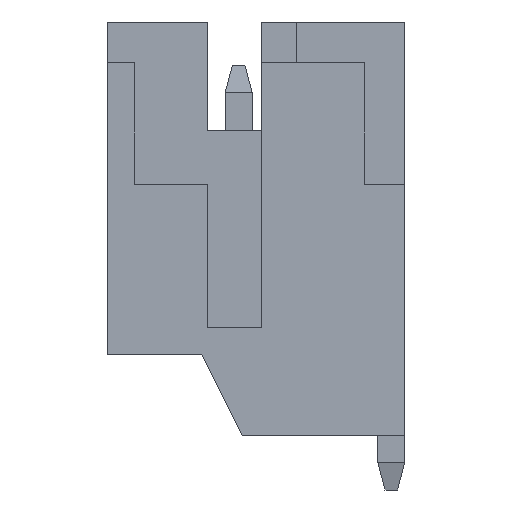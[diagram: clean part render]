
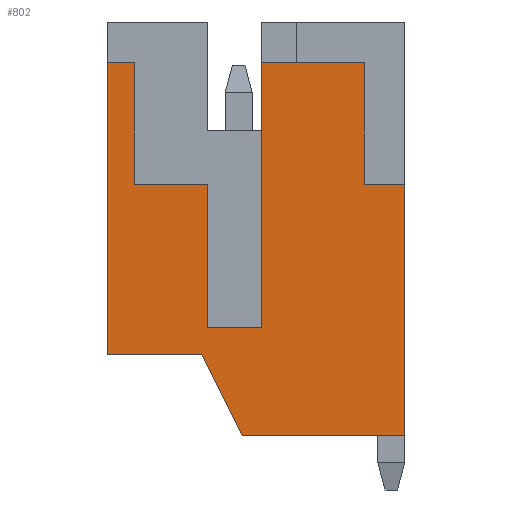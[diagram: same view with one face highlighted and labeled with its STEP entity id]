
A CAD part, left-side view. The second image highlights one B-rep face of the part: STEP entity #802.
In plain terms, the highlighted planar face has unit normal (-1, 0, 0).
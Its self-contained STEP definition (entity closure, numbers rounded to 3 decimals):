
#33 = LINE ( 'NONE', #486, #3350 ) ;
#57 = ORIENTED_EDGE ( 'NONE', *, *, #818, .F. ) ;
#66 = LINE ( 'NONE', #4594, #2860 ) ;
#202 = CARTESIAN_POINT ( 'NONE',  ( -3., 1.93, 5.4 ) ) ;
#237 = EDGE_LOOP ( 'NONE', ( #774, #1345, #1196, #2845, #3341, #2224, #549, #3415, #449, #1396, #1850, #57, #3068, #2094 ) ) ;
#280 = LINE ( 'NONE', #2753, #3090 ) ;
#297 = VERTEX_POINT ( 'NONE', #1133 ) ;
#317 = PLANE ( 'NONE',  #3844 ) ;
#449 = ORIENTED_EDGE ( 'NONE', *, *, #2692, .T. ) ;
#486 = CARTESIAN_POINT ( 'NONE',  ( -3., -0.42, 3.15 ) ) ;
#506 = EDGE_CURVE ( 'NONE', #2816, #3251, #66, .T. ) ;
#549 = ORIENTED_EDGE ( 'NONE', *, *, #1288, .F. ) ;
#567 = EDGE_CURVE ( 'NONE', #297, #2436, #4172, .T. ) ;
#638 = VERTEX_POINT ( 'NONE', #2404 ) ;
#639 = DIRECTION ( 'NONE',  ( 0., -1., 0. ) ) ;
#677 = VERTEX_POINT ( 'NONE', #3921 ) ;
#688 = EDGE_CURVE ( 'NONE', #4280, #1674, #4513, .T. ) ;
#707 = VERTEX_POINT ( 'NONE', #3937 ) ;
#709 = CARTESIAN_POINT ( 'NONE',  ( -3., 0.68, 0. ) ) ;
#731 = DIRECTION ( 'NONE',  ( -1., 0., 0. ) ) ;
#774 = ORIENTED_EDGE ( 'NONE', *, *, #688, .T. ) ;
#795 = VECTOR ( 'NONE', #3804, 1000. ) ;
#802 = ADVANCED_FACE ( 'NONE', ( #1606 ), #317, .T. ) ;
#818 = EDGE_CURVE ( 'NONE', #2758, #677, #2747, .T. ) ;
#819 = VERTEX_POINT ( 'NONE', #4716 ) ;
#901 = DIRECTION ( 'NONE',  ( 0., 0., 1. ) ) ;
#972 = LINE ( 'NONE', #1584, #1324 ) ;
#1048 = CARTESIAN_POINT ( 'NONE',  ( -3., -3.07, 5.4 ) ) ;
#1133 = CARTESIAN_POINT ( 'NONE',  ( -3., -0.42, 5.4 ) ) ;
#1196 = ORIENTED_EDGE ( 'NONE', *, *, #1969, .T. ) ;
#1211 = VECTOR ( 'NONE', #2180, 1000. ) ;
#1288 = EDGE_CURVE ( 'NONE', #819, #3251, #2928, .T. ) ;
#1324 = VECTOR ( 'NONE', #1973, 1000. ) ;
#1335 = CARTESIAN_POINT ( 'NONE',  ( -3., -3.07, -1.5 ) ) ;
#1345 = ORIENTED_EDGE ( 'NONE', *, *, #2744, .T. ) ;
#1355 = VERTEX_POINT ( 'NONE', #3945 ) ;
#1380 = DIRECTION ( 'NONE',  ( 0., 1., 0. ) ) ;
#1396 = ORIENTED_EDGE ( 'NONE', *, *, #567, .T. ) ;
#1452 = CARTESIAN_POINT ( 'NONE',  ( -3., -0.42, 0.5 ) ) ;
#1479 = CARTESIAN_POINT ( 'NONE',  ( -3., 0.58, 3.15 ) ) ;
#1492 = DIRECTION ( 'NONE',  ( 0., 0., 1. ) ) ;
#1498 = VECTOR ( 'NONE', #4451, 1000. ) ;
#1584 = CARTESIAN_POINT ( 'NONE',  ( -3., -0.42, 0.5 ) ) ;
#1606 = FACE_OUTER_BOUND ( 'NONE', #237, .T. ) ;
#1674 = VERTEX_POINT ( 'NONE', #3784 ) ;
#1850 = ORIENTED_EDGE ( 'NONE', *, *, #2084, .F. ) ;
#1875 = VERTEX_POINT ( 'NONE', #709 ) ;
#1893 = EDGE_CURVE ( 'NONE', #707, #4280, #1959, .T. ) ;
#1898 = LINE ( 'NONE', #2976, #1498 ) ;
#1899 = EDGE_CURVE ( 'NONE', #1875, #638, #1898, .T. ) ;
#1959 = LINE ( 'NONE', #3677, #2855 ) ;
#1969 = EDGE_CURVE ( 'NONE', #1355, #1875, #2918, .T. ) ;
#1973 = DIRECTION ( 'NONE',  ( 0., -1., 0. ) ) ;
#1994 = EDGE_CURVE ( 'NONE', #819, #2761, #2241, .T. ) ;
#2038 = DIRECTION ( 'NONE',  ( 0., -1., 0. ) ) ;
#2072 = VECTOR ( 'NONE', #2038, 1000. ) ;
#2084 = EDGE_CURVE ( 'NONE', #677, #2436, #972, .T. ) ;
#2094 = ORIENTED_EDGE ( 'NONE', *, *, #1893, .T. ) ;
#2165 = EDGE_CURVE ( 'NONE', #638, #2816, #3093, .T. ) ;
#2180 = DIRECTION ( 'NONE',  ( 0., 0., -1. ) ) ;
#2191 = VECTOR ( 'NONE', #639, 1000. ) ;
#2224 = ORIENTED_EDGE ( 'NONE', *, *, #506, .T. ) ;
#2231 = LINE ( 'NONE', #2748, #795 ) ;
#2241 = LINE ( 'NONE', #2259, #4057 ) ;
#2259 = CARTESIAN_POINT ( 'NONE',  ( -3., -2.32, 3.15 ) ) ;
#2404 = CARTESIAN_POINT ( 'NONE',  ( -3., -0.07, -1.5 ) ) ;
#2436 = VERTEX_POINT ( 'NONE', #1452 ) ;
#2692 = EDGE_CURVE ( 'NONE', #2761, #297, #2231, .T. ) ;
#2744 = EDGE_CURVE ( 'NONE', #1674, #1355, #280, .T. ) ;
#2747 = LINE ( 'NONE', #1479, #1211 ) ;
#2748 = CARTESIAN_POINT ( 'NONE',  ( -3., -3.07, 5.4 ) ) ;
#2753 = CARTESIAN_POINT ( 'NONE',  ( -3., 2.43, 6.15 ) ) ;
#2758 = VERTEX_POINT ( 'NONE', #2919 ) ;
#2761 = VERTEX_POINT ( 'NONE', #4618 ) ;
#2807 = DIRECTION ( 'NONE',  ( 0., 0., -1. ) ) ;
#2816 = VERTEX_POINT ( 'NONE', #1335 ) ;
#2829 = CARTESIAN_POINT ( 'NONE',  ( -3., -2.32, 3.15 ) ) ;
#2845 = ORIENTED_EDGE ( 'NONE', *, *, #1899, .T. ) ;
#2855 = VECTOR ( 'NONE', #1492, 1000. ) ;
#2860 = VECTOR ( 'NONE', #901, 1000. ) ;
#2918 = LINE ( 'NONE', #2954, #3208 ) ;
#2919 = CARTESIAN_POINT ( 'NONE',  ( -3., 0.58, 3.15 ) ) ;
#2928 = LINE ( 'NONE', #2829, #2191 ) ;
#2954 = CARTESIAN_POINT ( 'NONE',  ( -3., 2.43, 0. ) ) ;
#2976 = CARTESIAN_POINT ( 'NONE',  ( -3., -0.07, -1.5 ) ) ;
#3068 = ORIENTED_EDGE ( 'NONE', *, *, #4084, .F. ) ;
#3090 = VECTOR ( 'NONE', #2807, 1000. ) ;
#3093 = LINE ( 'NONE', #4254, #2072 ) ;
#3208 = VECTOR ( 'NONE', #3699, 1000. ) ;
#3251 = VERTEX_POINT ( 'NONE', #4030 ) ;
#3341 = ORIENTED_EDGE ( 'NONE', *, *, #2165, .T. ) ;
#3349 = DIRECTION ( 'NONE',  ( 0., -1., 0. ) ) ;
#3350 = VECTOR ( 'NONE', #3349, 1000. ) ;
#3415 = ORIENTED_EDGE ( 'NONE', *, *, #1994, .T. ) ;
#3539 = VECTOR ( 'NONE', #1380, 1000. ) ;
#3614 = DIRECTION ( 'NONE',  ( 0., -1., 0. ) ) ;
#3677 = CARTESIAN_POINT ( 'NONE',  ( -3., 1.93, 3.15 ) ) ;
#3699 = DIRECTION ( 'NONE',  ( 0., -1., 0. ) ) ;
#3777 = DIRECTION ( 'NONE',  ( 0., 0., 1. ) ) ;
#3784 = CARTESIAN_POINT ( 'NONE',  ( -3., 2.43, 5.4 ) ) ;
#3804 = DIRECTION ( 'NONE',  ( 0., 1., 0. ) ) ;
#3813 = CARTESIAN_POINT ( 'NONE',  ( -3., -0.42, 6.15 ) ) ;
#3844 = AXIS2_PLACEMENT_3D ( 'NONE', #4323, #731, #3614 ) ;
#3874 = DIRECTION ( 'NONE',  ( 0., 0., -1. ) ) ;
#3921 = CARTESIAN_POINT ( 'NONE',  ( -3., 0.58, 0.5 ) ) ;
#3937 = CARTESIAN_POINT ( 'NONE',  ( -3., 1.93, 3.15 ) ) ;
#3945 = CARTESIAN_POINT ( 'NONE',  ( -3., 2.43, 0. ) ) ;
#4030 = CARTESIAN_POINT ( 'NONE',  ( -3., -3.07, 3.15 ) ) ;
#4057 = VECTOR ( 'NONE', #3777, 1000. ) ;
#4084 = EDGE_CURVE ( 'NONE', #707, #2758, #33, .T. ) ;
#4172 = LINE ( 'NONE', #3813, #4622 ) ;
#4254 = CARTESIAN_POINT ( 'NONE',  ( -3., -3.07, -1.5 ) ) ;
#4280 = VERTEX_POINT ( 'NONE', #202 ) ;
#4323 = CARTESIAN_POINT ( 'NONE',  ( -3., 0., 0. ) ) ;
#4451 = DIRECTION ( 'NONE',  ( 0., -0.447, -0.894 ) ) ;
#4513 = LINE ( 'NONE', #1048, #3539 ) ;
#4594 = CARTESIAN_POINT ( 'NONE',  ( -3., -3.07, 6.15 ) ) ;
#4618 = CARTESIAN_POINT ( 'NONE',  ( -3., -2.32, 5.4 ) ) ;
#4622 = VECTOR ( 'NONE', #3874, 1000. ) ;
#4716 = CARTESIAN_POINT ( 'NONE',  ( -3., -2.32, 3.15 ) ) ;
